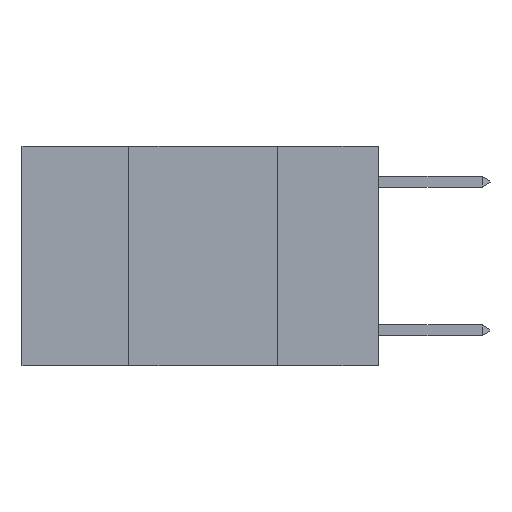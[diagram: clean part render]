
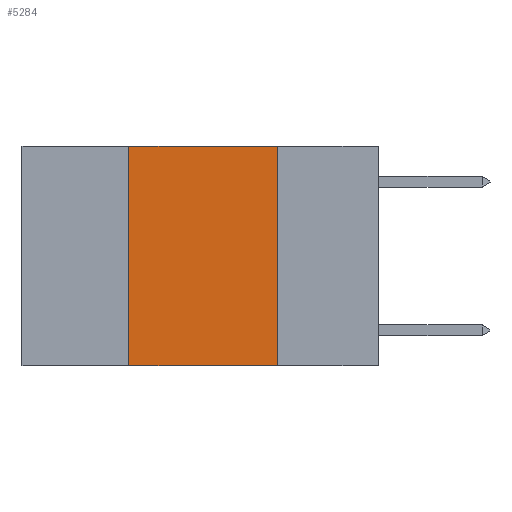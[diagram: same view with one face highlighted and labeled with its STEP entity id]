
A CAD part, left-side view. The second image highlights one B-rep face of the part: STEP entity #5284.
In plain terms, the highlighted planar face has unit normal (-1, 0, 0).
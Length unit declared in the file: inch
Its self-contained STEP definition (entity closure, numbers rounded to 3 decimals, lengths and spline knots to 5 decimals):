
#593 = DIRECTION ( 'NONE',  ( 0., -1., 0. ) ) ;
#773 = CARTESIAN_POINT ( 'NONE',  ( 0., 0.6, -0.37 ) ) ;
#978 = DIRECTION ( 'NONE',  ( 0., 0., -1. ) ) ;
#980 = DIRECTION ( 'NONE',  ( 1., 0., 0. ) ) ;
#994 = CARTESIAN_POINT ( 'NONE',  ( 0., 0.6, 0. ) ) ;
#1237 = PLANE ( 'NONE',  #4033 ) ;
#1671 = VERTEX_POINT ( 'NONE', #7005 ) ;
#2025 = EDGE_CURVE ( 'NONE', #1671, #5895, #8879, .T. ) ;
#2688 = DIRECTION ( 'NONE',  ( 0., -1., 0. ) ) ;
#2761 = CARTESIAN_POINT ( 'NONE',  ( 0., 0.6, 0. ) ) ;
#3419 = VECTOR ( 'NONE', #8450, 39.37008 ) ;
#3462 = LINE ( 'NONE', #7580, #3419 ) ;
#3946 = VECTOR ( 'NONE', #4105, 39.37008 ) ;
#3955 = LINE ( 'NONE', #4102, #3946 ) ;
#4029 = CARTESIAN_POINT ( 'NONE',  ( 0., 0.17, 0. ) ) ;
#4033 = AXIS2_PLACEMENT_3D ( 'NONE', #994, #980, #978 ) ;
#4042 = ORIENTED_EDGE ( 'NONE', *, *, #9033, .F. ) ;
#4102 = CARTESIAN_POINT ( 'NONE',  ( 0., 0.17, 0. ) ) ;
#4105 = DIRECTION ( 'NONE',  ( 0., 0., -1. ) ) ;
#4207 = ORIENTED_EDGE ( 'NONE', *, *, #7943, .F. ) ;
#4297 = CARTESIAN_POINT ( 'NONE',  ( 0., 0.17, -0.37 ) ) ;
#4987 = ORIENTED_EDGE ( 'NONE', *, *, #2025, .T. ) ;
#5284 = ADVANCED_FACE ( 'NONE', ( #8590 ), #1237, .F. ) ;
#5493 = ORIENTED_EDGE ( 'NONE', *, *, #9227, .F. ) ;
#5895 = VERTEX_POINT ( 'NONE', #4297 ) ;
#6398 = LINE ( 'NONE', #2761, #6424 ) ;
#6424 = VECTOR ( 'NONE', #2688, 39.37008 ) ;
#6584 = CARTESIAN_POINT ( 'NONE',  ( 0., 0.42, 0. ) ) ;
#7005 = CARTESIAN_POINT ( 'NONE',  ( 0., 0.42, -0.37 ) ) ;
#7422 = VERTEX_POINT ( 'NONE', #6584 ) ;
#7580 = CARTESIAN_POINT ( 'NONE',  ( 0., 0.42, 0. ) ) ;
#7786 = VERTEX_POINT ( 'NONE', #4029 ) ;
#7943 = EDGE_CURVE ( 'NONE', #7422, #7786, #6398, .T. ) ;
#8450 = DIRECTION ( 'NONE',  ( 0., 0., 1. ) ) ;
#8590 = FACE_OUTER_BOUND ( 'NONE', #9790, .T. ) ;
#8804 = VECTOR ( 'NONE', #593, 39.37008 ) ;
#8879 = LINE ( 'NONE', #773, #8804 ) ;
#9033 = EDGE_CURVE ( 'NONE', #7786, #5895, #3955, .T. ) ;
#9227 = EDGE_CURVE ( 'NONE', #1671, #7422, #3462, .T. ) ;
#9790 = EDGE_LOOP ( 'NONE', ( #4042, #4207, #5493, #4987 ) ) ;
